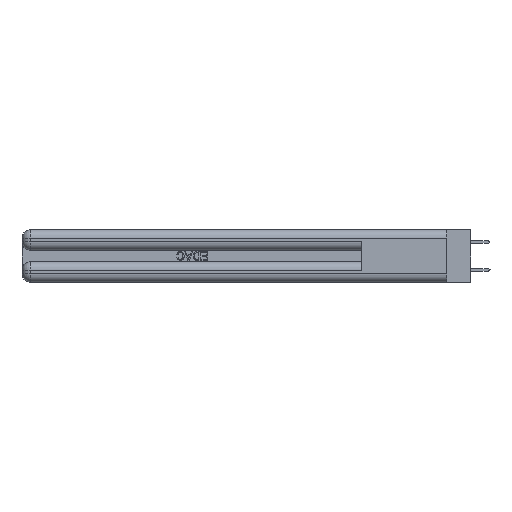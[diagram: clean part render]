
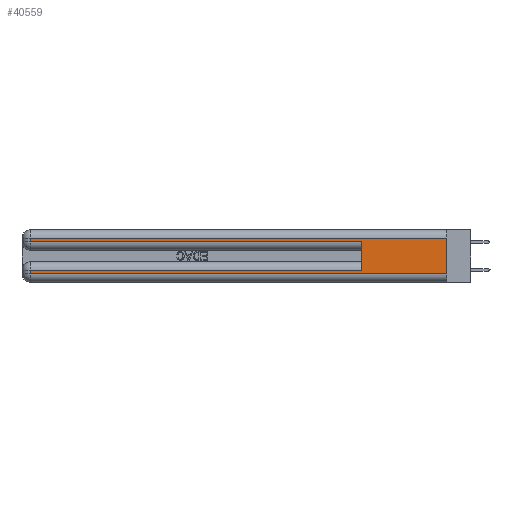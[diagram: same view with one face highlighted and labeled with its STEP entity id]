
A CAD part, left-side view. The second image highlights one B-rep face of the part: STEP entity #40559.
In plain terms, the highlighted planar face has unit normal (-1, 0, 0).
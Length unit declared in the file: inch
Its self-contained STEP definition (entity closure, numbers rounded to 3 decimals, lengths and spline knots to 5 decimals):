
#382 = DIRECTION ( 'NONE',  ( 0., -1., 0. ) ) ;
#1796 = VECTOR ( 'NONE', #382, 39.37008 ) ;
#2201 = EDGE_CURVE ( 'NONE', #29945, #27035, #31796, .T. ) ;
#2783 = VERTEX_POINT ( 'NONE', #23752 ) ;
#2837 = EDGE_CURVE ( 'NONE', #17483, #11042, #4534, .T. ) ;
#4534 = LINE ( 'NONE', #34050, #18667 ) ;
#4989 = VECTOR ( 'NONE', #29182, 39.37008 ) ;
#5074 = CARTESIAN_POINT ( 'NONE',  ( 0., 0., 0.085 ) ) ;
#5684 = LINE ( 'NONE', #31991, #38929 ) ;
#5915 = CARTESIAN_POINT ( 'NONE',  ( 0., 2.94, 0.37 ) ) ;
#7785 = VECTOR ( 'NONE', #20684, 39.37008 ) ;
#7966 = ORIENTED_EDGE ( 'NONE', *, *, #25874, .T. ) ;
#9402 = CARTESIAN_POINT ( 'NONE',  ( 0., 2.94, 0.06 ) ) ;
#11042 = VERTEX_POINT ( 'NONE', #40750 ) ;
#12011 = DIRECTION ( 'NONE',  ( 1., 0., 0. ) ) ;
#12161 = VERTEX_POINT ( 'NONE', #21619 ) ;
#14260 = VERTEX_POINT ( 'NONE', #39487 ) ;
#14489 = LINE ( 'NONE', #5074, #28971 ) ;
#15456 = PLANE ( 'NONE',  #18535 ) ;
#15672 = FACE_OUTER_BOUND ( 'NONE', #28811, .T. ) ;
#16023 = EDGE_CURVE ( 'NONE', #20577, #29945, #20313, .T. ) ;
#16611 = LINE ( 'NONE', #25814, #1796 ) ;
#17483 = VERTEX_POINT ( 'NONE', #9402 ) ;
#17801 = ORIENTED_EDGE ( 'NONE', *, *, #25894, .T. ) ;
#18373 = DIRECTION ( 'NONE',  ( 0., 0., 1. ) ) ;
#18393 = EDGE_CURVE ( 'NONE', #20577, #11042, #5684, .T. ) ;
#18535 = AXIS2_PLACEMENT_3D ( 'NONE', #21615, #12011, #34706 ) ;
#18667 = VECTOR ( 'NONE', #20771, 39.37008 ) ;
#20313 = LINE ( 'NONE', #33367, #28499 ) ;
#20577 = VERTEX_POINT ( 'NONE', #41206 ) ;
#20684 = DIRECTION ( 'NONE',  ( 0., 0., -1. ) ) ;
#20737 = CARTESIAN_POINT ( 'NONE',  ( 0., 2.94, 0.285 ) ) ;
#20771 = DIRECTION ( 'NONE',  ( 0., -1., 0. ) ) ;
#21615 = CARTESIAN_POINT ( 'NONE',  ( 0., 0., 0.37 ) ) ;
#21619 = CARTESIAN_POINT ( 'NONE',  ( 0., 0.6, 0.085 ) ) ;
#23660 = CARTESIAN_POINT ( 'NONE',  ( 0., 2.94, 0.37 ) ) ;
#23752 = CARTESIAN_POINT ( 'NONE',  ( 0., 2.94, 0.085 ) ) ;
#25434 = LINE ( 'NONE', #38735, #27044 ) ;
#25814 = CARTESIAN_POINT ( 'NONE',  ( 0., 0., 0.285 ) ) ;
#25874 = EDGE_CURVE ( 'NONE', #12161, #2783, #14489, .T. ) ;
#25894 = EDGE_CURVE ( 'NONE', #2783, #17483, #34171, .T. ) ;
#25997 = ORIENTED_EDGE ( 'NONE', *, *, #16023, .T. ) ;
#27035 = VERTEX_POINT ( 'NONE', #20737 ) ;
#27044 = VECTOR ( 'NONE', #18373, 39.37008 ) ;
#27460 = ORIENTED_EDGE ( 'NONE', *, *, #31097, .F. ) ;
#28499 = VECTOR ( 'NONE', #40475, 39.37008 ) ;
#28811 = EDGE_LOOP ( 'NONE', ( #41555, #25997, #38347, #35870, #27460, #7966, #17801, #40016 ) ) ;
#28971 = VECTOR ( 'NONE', #39996, 39.37008 ) ;
#29182 = DIRECTION ( 'NONE',  ( 0., 0., -1. ) ) ;
#29945 = VERTEX_POINT ( 'NONE', #31860 ) ;
#31097 = EDGE_CURVE ( 'NONE', #12161, #14260, #25434, .T. ) ;
#31796 = LINE ( 'NONE', #5915, #4989 ) ;
#31860 = CARTESIAN_POINT ( 'NONE',  ( 0., 2.94, 0.31 ) ) ;
#31991 = CARTESIAN_POINT ( 'NONE',  ( 0., 0., 0.37 ) ) ;
#32687 = EDGE_CURVE ( 'NONE', #27035, #14260, #16611, .T. ) ;
#33367 = CARTESIAN_POINT ( 'NONE',  ( 0., 0., 0.31 ) ) ;
#34050 = CARTESIAN_POINT ( 'NONE',  ( 0., 0., 0.06 ) ) ;
#34171 = LINE ( 'NONE', #23660, #7785 ) ;
#34706 = DIRECTION ( 'NONE',  ( 0., 0., -1. ) ) ;
#35621 = DIRECTION ( 'NONE',  ( 0., 0., -1. ) ) ;
#35870 = ORIENTED_EDGE ( 'NONE', *, *, #32687, .T. ) ;
#38347 = ORIENTED_EDGE ( 'NONE', *, *, #2201, .T. ) ;
#38735 = CARTESIAN_POINT ( 'NONE',  ( 0., 0.6, 0.145 ) ) ;
#38929 = VECTOR ( 'NONE', #35621, 39.37008 ) ;
#39487 = CARTESIAN_POINT ( 'NONE',  ( 0., 0.6, 0.285 ) ) ;
#39996 = DIRECTION ( 'NONE',  ( 0., 1., 0. ) ) ;
#40016 = ORIENTED_EDGE ( 'NONE', *, *, #2837, .T. ) ;
#40475 = DIRECTION ( 'NONE',  ( 0., 1., 0. ) ) ;
#40559 = ADVANCED_FACE ( 'NONE', ( #15672 ), #15456, .F. ) ;
#40750 = CARTESIAN_POINT ( 'NONE',  ( 0., 0., 0.06 ) ) ;
#41206 = CARTESIAN_POINT ( 'NONE',  ( 0., 0., 0.31 ) ) ;
#41555 = ORIENTED_EDGE ( 'NONE', *, *, #18393, .F. ) ;
